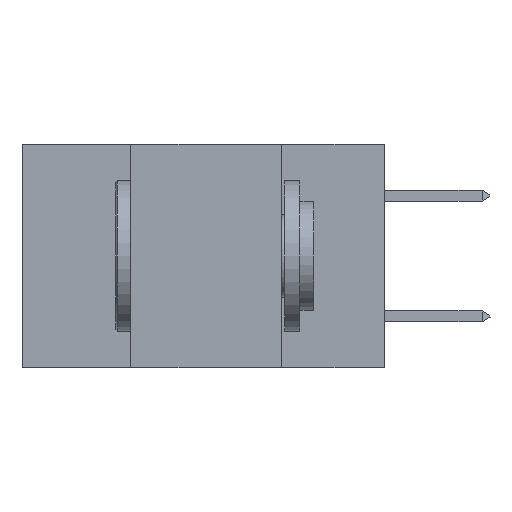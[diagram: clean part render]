
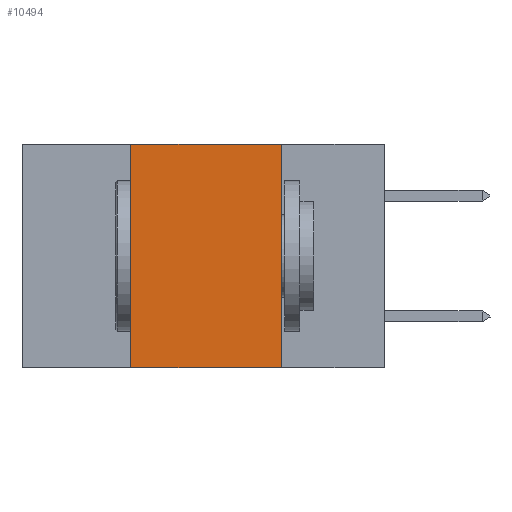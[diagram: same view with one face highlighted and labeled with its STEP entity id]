
A CAD part, left-side view. The second image highlights one B-rep face of the part: STEP entity #10494.
In plain terms, the highlighted planar face has unit normal (-1, 0, 0).
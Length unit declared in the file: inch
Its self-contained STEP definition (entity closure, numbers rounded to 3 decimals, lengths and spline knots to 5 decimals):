
#337 = ORIENTED_EDGE ( 'NONE', *, *, #11004, .F. ) ;
#878 = EDGE_LOOP ( 'NONE', ( #9603, #337, #5302, #4568 ) ) ;
#940 = DIRECTION ( 'NONE',  ( 0., 0., -1. ) ) ;
#1448 = CARTESIAN_POINT ( 'NONE',  ( 0., 0.42, 0. ) ) ;
#2003 = CARTESIAN_POINT ( 'NONE',  ( 0., 0.17, -0.37 ) ) ;
#2346 = LINE ( 'NONE', #12667, #6261 ) ;
#2486 = DIRECTION ( 'NONE',  ( 0., 0., 1. ) ) ;
#2732 = VECTOR ( 'NONE', #7517, 39.37008 ) ;
#3281 = DIRECTION ( 'NONE',  ( 0., 0., -1. ) ) ;
#3303 = VECTOR ( 'NONE', #3281, 39.37008 ) ;
#3402 = PLANE ( 'NONE',  #4660 ) ;
#4173 = DIRECTION ( 'NONE',  ( 0., -1., 0. ) ) ;
#4568 = ORIENTED_EDGE ( 'NONE', *, *, #10732, .T. ) ;
#4660 = AXIS2_PLACEMENT_3D ( 'NONE', #16060, #13631, #940 ) ;
#5256 = CARTESIAN_POINT ( 'NONE',  ( 0., 0.42, -0.37 ) ) ;
#5302 = ORIENTED_EDGE ( 'NONE', *, *, #15381, .F. ) ;
#6261 = VECTOR ( 'NONE', #4173, 39.37008 ) ;
#6807 = CARTESIAN_POINT ( 'NONE',  ( 0., 0.17, 0. ) ) ;
#7201 = EDGE_CURVE ( 'NONE', #12399, #12541, #9958, .T. ) ;
#7517 = DIRECTION ( 'NONE',  ( 0., -1., 0. ) ) ;
#9603 = ORIENTED_EDGE ( 'NONE', *, *, #7201, .F. ) ;
#9958 = LINE ( 'NONE', #12041, #3303 ) ;
#10039 = VERTEX_POINT ( 'NONE', #5256 ) ;
#10494 = ADVANCED_FACE ( 'NONE', ( #13053 ), #3402, .F. ) ;
#10732 = EDGE_CURVE ( 'NONE', #10039, #12541, #10794, .T. ) ;
#10766 = VERTEX_POINT ( 'NONE', #1448 ) ;
#10794 = LINE ( 'NONE', #11351, #2732 ) ;
#11004 = EDGE_CURVE ( 'NONE', #10766, #12399, #2346, .T. ) ;
#11237 = LINE ( 'NONE', #11452, #13853 ) ;
#11351 = CARTESIAN_POINT ( 'NONE',  ( 0., 0.6, -0.37 ) ) ;
#11452 = CARTESIAN_POINT ( 'NONE',  ( 0., 0.42, 0. ) ) ;
#12041 = CARTESIAN_POINT ( 'NONE',  ( 0., 0.17, 0. ) ) ;
#12399 = VERTEX_POINT ( 'NONE', #6807 ) ;
#12541 = VERTEX_POINT ( 'NONE', #2003 ) ;
#12667 = CARTESIAN_POINT ( 'NONE',  ( 0., 0.6, 0. ) ) ;
#13053 = FACE_OUTER_BOUND ( 'NONE', #878, .T. ) ;
#13631 = DIRECTION ( 'NONE',  ( 1., 0., 0. ) ) ;
#13853 = VECTOR ( 'NONE', #2486, 39.37008 ) ;
#15381 = EDGE_CURVE ( 'NONE', #10039, #10766, #11237, .T. ) ;
#16060 = CARTESIAN_POINT ( 'NONE',  ( 0., 0.6, 0. ) ) ;
